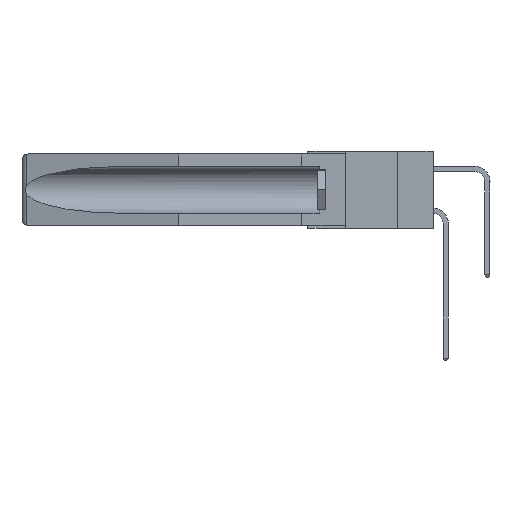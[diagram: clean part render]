
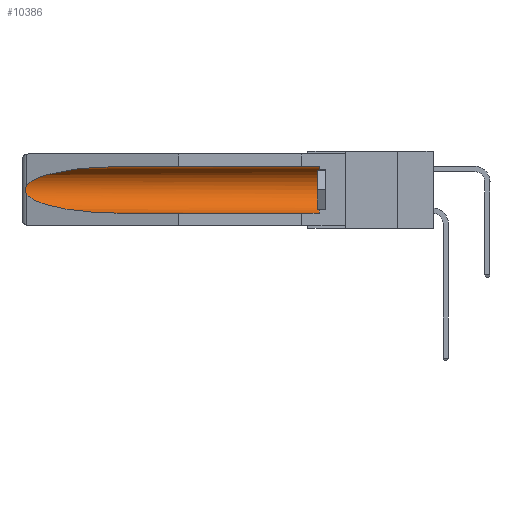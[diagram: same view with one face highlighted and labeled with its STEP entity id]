
A CAD part, left-side view. The second image highlights one B-rep face of the part: STEP entity #10386.
In plain terms, the highlighted cylindrical face has radius 2.857 mm (diameter 5.715 mm), a partial arc.
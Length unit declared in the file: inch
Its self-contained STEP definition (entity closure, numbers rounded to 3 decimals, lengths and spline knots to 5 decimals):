
#2 = B_SPLINE_CURVE_WITH_KNOTS ( 'NONE', 3,
 ( #7754, #12825, #8831, #16498, #18457, #7873, #17506, #12932, #4689, #10223 ),
 .UNSPECIFIED., .F., .F.,
 ( 4, 2, 2, 2, 4 ),
 ( 0., 0.00029, 0.00058, 0.00087, 0.00117 ),
 .UNSPECIFIED. ) ;
#81 = CIRCLE ( 'NONE', #13340, 0.1125 ) ;
#418 = VECTOR ( 'NONE', #18829, 39.37008 ) ;
#467 = DIRECTION ( 'NONE',  ( 0., 1., 0. ) ) ;
#589 = ORIENTED_EDGE ( 'NONE', *, *, #14797, .F. ) ;
#670 = CARTESIAN_POINT ( 'NONE',  ( 0.155, 1.07973, -0.284 ) ) ;
#1727 = DIRECTION ( 'NONE',  ( 0., 0., 1. ) ) ;
#2070 = VERTEX_POINT ( 'NONE', #4313 ) ;
#2220 = CARTESIAN_POINT ( 'NONE',  ( 0.155, -0.30754, -0.284 ) ) ;
#2545 = CARTESIAN_POINT ( 'NONE',  ( 0.155, -0.30754, -0.1715 ) ) ;
#2607 = DIRECTION ( 'NONE',  ( 0., 0., 1. ) ) ;
#2874 = CARTESIAN_POINT ( 'NONE',  ( 0.155, 0.126, -0.284 ) ) ;
#4313 = CARTESIAN_POINT ( 'NONE',  ( 0.155, 1.07973, -0.059 ) ) ;
#4689 = CARTESIAN_POINT ( 'NONE',  ( 0.26597, 1.5296, -0.19026 ) ) ;
#5184 = CARTESIAN_POINT ( 'NONE',  ( 0.21114, 1.30732, -0.284 ) ) ;
#5517 = AXIS2_PLACEMENT_3D ( 'NONE', #2545, #16595, #1727 ) ;
#6674 = CARTESIAN_POINT ( 'NONE',  ( 0.155, -0.30754, -0.059 ) ) ;
#7562 = EDGE_CURVE ( 'NONE', #15770, #12662, #81, .T. ) ;
#7754 = CARTESIAN_POINT ( 'NONE',  ( 0.26537, 1.52718, -0.14972 ) ) ;
#7873 = CARTESIAN_POINT ( 'NONE',  ( 0.2675, 1.53308, -0.17534 ) ) ;
#8187 = CARTESIAN_POINT ( 'NONE',  ( 0.26537, 1.52718, -0.19328 ) ) ;
#8496 = VERTEX_POINT ( 'NONE', #9323 ) ;
#8497 = DIRECTION ( 'NONE',  ( 0., -1., 0. ) ) ;
#8719 = LINE ( 'NONE', #6674, #418 ) ;
#8831 = CARTESIAN_POINT ( 'NONE',  ( 0.26654, 1.53092, -0.15636 ) ) ;
#8940 = CARTESIAN_POINT ( 'NONE',  ( 0.26537, 1.52718, -0.14972 ) ) ;
#9323 = CARTESIAN_POINT ( 'NONE',  ( 0.26537, 1.52718, -0.14972 ) ) ;
#9372 = EDGE_CURVE ( 'NONE', #12662, #2070, #8719, .T. ) ;
#10223 = CARTESIAN_POINT ( 'NONE',  ( 0.26537, 1.52718, -0.19328 ) ) ;
#10271 =( BOUNDED_CURVE ( )  B_SPLINE_CURVE ( 3, ( #8187, #19057, #5184, #670 ),
 .UNSPECIFIED., .F., .T. ) 
 B_SPLINE_CURVE_WITH_KNOTS ( ( 4, 4 ),
 ( 0.1948, 1.5708 ),
 .UNSPECIFIED. ) 
 CURVE ( )  GEOMETRIC_REPRESENTATION_ITEM ( )  RATIONAL_B_SPLINE_CURVE ( ( 1., 0.848, 0.848, 1. ) ) 
 REPRESENTATION_ITEM ( '' )  );
#10386 = ADVANCED_FACE ( 'NONE', ( #17656 ), #10629, .F. ) ;
#10629 = CYLINDRICAL_SURFACE ( 'NONE', #5517, 0.1125 ) ;
#11106 = EDGE_CURVE ( 'NONE', #8496, #18878, #2, .T. ) ;
#11137 = ORIENTED_EDGE ( 'NONE', *, *, #14262, .T. ) ;
#12662 = VERTEX_POINT ( 'NONE', #13912 ) ;
#12825 = CARTESIAN_POINT ( 'NONE',  ( 0.26597, 1.52961, -0.15275 ) ) ;
#12932 = CARTESIAN_POINT ( 'NONE',  ( 0.26655, 1.53094, -0.18657 ) ) ;
#13340 = AXIS2_PLACEMENT_3D ( 'NONE', #14710, #8497, #2607 ) ;
#13353 = EDGE_CURVE ( 'NONE', #2070, #8496, #14517, .T. ) ;
#13667 = CARTESIAN_POINT ( 'NONE',  ( 0.25451, 1.48313, -0.09465 ) ) ;
#13683 = VERTEX_POINT ( 'NONE', #17982 ) ;
#13912 = CARTESIAN_POINT ( 'NONE',  ( 0.155, 0.126, -0.059 ) ) ;
#14046 = LINE ( 'NONE', #2220, #15973 ) ;
#14262 = EDGE_CURVE ( 'NONE', #18878, #13683, #10271, .T. ) ;
#14517 =( BOUNDED_CURVE ( )  B_SPLINE_CURVE ( 3, ( #15146, #16878, #13667, #8940 ),
 .UNSPECIFIED., .F., .F. ) 
 B_SPLINE_CURVE_WITH_KNOTS ( ( 4, 4 ),
 ( 4.71239, 6.08839 ),
 .UNSPECIFIED. ) 
 CURVE ( )  GEOMETRIC_REPRESENTATION_ITEM ( )  RATIONAL_B_SPLINE_CURVE ( ( 1., 0.848, 0.848, 1. ) ) 
 REPRESENTATION_ITEM ( '' )  );
#14710 = CARTESIAN_POINT ( 'NONE',  ( 0.155, 0.126, -0.1715 ) ) ;
#14797 = EDGE_CURVE ( 'NONE', #15770, #13683, #14046, .T. ) ;
#15146 = CARTESIAN_POINT ( 'NONE',  ( 0.155, 1.07973, -0.059 ) ) ;
#15770 = VERTEX_POINT ( 'NONE', #2874 ) ;
#15973 = VECTOR ( 'NONE', #467, 39.37008 ) ;
#16122 = EDGE_LOOP ( 'NONE', ( #17079, #19508, #11137, #589, #19580, #18261 ) ) ;
#16498 = CARTESIAN_POINT ( 'NONE',  ( 0.2673, 1.5327, -0.16383 ) ) ;
#16595 = DIRECTION ( 'NONE',  ( 0., 1., 0. ) ) ;
#16878 = CARTESIAN_POINT ( 'NONE',  ( 0.21114, 1.30732, -0.059 ) ) ;
#17079 = ORIENTED_EDGE ( 'NONE', *, *, #13353, .T. ) ;
#17416 = CARTESIAN_POINT ( 'NONE',  ( 0.26537, 1.52718, -0.19328 ) ) ;
#17506 = CARTESIAN_POINT ( 'NONE',  ( 0.2673, 1.53269, -0.17917 ) ) ;
#17656 = FACE_OUTER_BOUND ( 'NONE', #16122, .T. ) ;
#17982 = CARTESIAN_POINT ( 'NONE',  ( 0.155, 1.07973, -0.284 ) ) ;
#18261 = ORIENTED_EDGE ( 'NONE', *, *, #9372, .T. ) ;
#18457 = CARTESIAN_POINT ( 'NONE',  ( 0.2675, 1.53308, -0.16763 ) ) ;
#18829 = DIRECTION ( 'NONE',  ( 0., 1., 0. ) ) ;
#18878 = VERTEX_POINT ( 'NONE', #17416 ) ;
#19057 = CARTESIAN_POINT ( 'NONE',  ( 0.25451, 1.48313, -0.24835 ) ) ;
#19508 = ORIENTED_EDGE ( 'NONE', *, *, #11106, .T. ) ;
#19580 = ORIENTED_EDGE ( 'NONE', *, *, #7562, .T. ) ;
